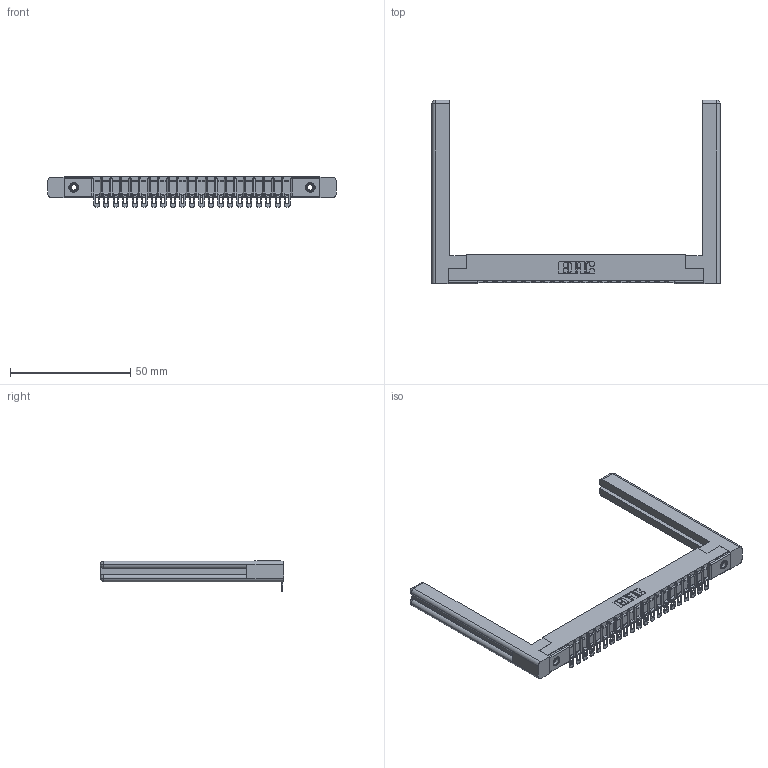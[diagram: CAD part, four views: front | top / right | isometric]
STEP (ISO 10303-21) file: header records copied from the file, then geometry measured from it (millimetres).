
FILE_DESCRIPTION (( 'STEP AP203' ), '1' );
FILE_NAME ('357-021-454-158.STEP', '2020-10-01T07:04:24', ( '' ), ( '' ), 'SwSTEP 2.0', 'SolidWorks 2020', '' );
FILE_SCHEMA (( 'CONFIG_CONTROL_DESIGN' ));
Length unit declared in the file: inch
Products named in the file (5): 357-021-454-158; 307-290-002_554; 307-220-058; 345-250-001_345-250-001-102; 307 Part_.156 Dia Mounting Holes
Assembly tree (26 placements, depth 2):
  357-021-454-158
    307 Part_.156 Dia Mounting Holes
    307-290-002_554  x21
    307-220-058  x2
    345-250-001_345-250-001-102  x2
Bounding box: 119.84 x 76.33 x 12.52 mm (x, y, z)
Volume: 15596.8 mm3; surface area: 19457.5 mm2
Topology: 26 solids, 26 shells, 1983 faces, 5990 edges, 3920 vertices
Faces by surface type: plane 1120, cylinder 795, sphere 44, torus 12, cone 12
Entity records: 24190 total; most frequent: CARTESIAN_POINT 4085, ORIENTED_EDGE 4014, DIRECTION 3945, EDGE_CURVE 2007, LINE 1517, VECTOR 1517, VERTEX_POINT 1300, AXIS2_PLACEMENT_3D 1214
